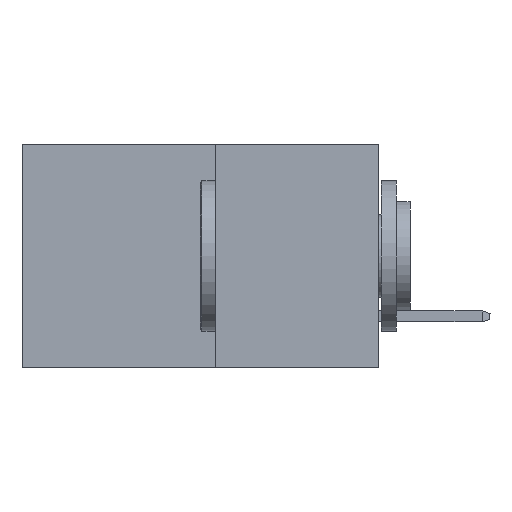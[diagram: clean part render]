
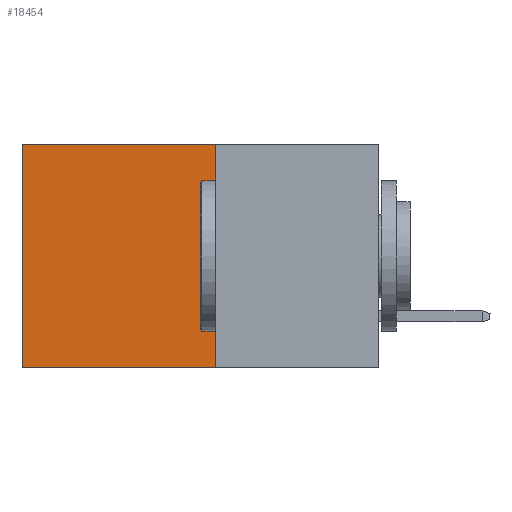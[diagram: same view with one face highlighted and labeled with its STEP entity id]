
A CAD part, left-side view. The second image highlights one B-rep face of the part: STEP entity #18454.
In plain terms, the highlighted planar face has unit normal (-1, 0, 0).
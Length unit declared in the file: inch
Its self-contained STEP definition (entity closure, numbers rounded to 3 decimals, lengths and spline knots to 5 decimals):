
#145 = CARTESIAN_POINT ( 'NONE',  ( 0.277, 0.59, -0.37 ) ) ;
#204 = VERTEX_POINT ( 'NONE', #19812 ) ;
#2008 = VECTOR ( 'NONE', #19218, 39.37008 ) ;
#2810 = LINE ( 'NONE', #18738, #2008 ) ;
#3067 = DIRECTION ( 'NONE',  ( 0., 0., -1. ) ) ;
#4759 = LINE ( 'NONE', #145, #11527 ) ;
#4954 = CARTESIAN_POINT ( 'NONE',  ( 0.277, 0.27, 0. ) ) ;
#6103 = ORIENTED_EDGE ( 'NONE', *, *, #27574, .F. ) ;
#7174 = ORIENTED_EDGE ( 'NONE', *, *, #7443, .T. ) ;
#7443 = EDGE_CURVE ( 'NONE', #14310, #204, #4759, .T. ) ;
#8168 = LINE ( 'NONE', #4954, #25371 ) ;
#8325 = CARTESIAN_POINT ( 'NONE',  ( 0.277, 0.59, 0. ) ) ;
#9046 = DIRECTION ( 'NONE',  ( 0., 1., 0. ) ) ;
#9050 = CARTESIAN_POINT ( 'NONE',  ( 0.277, 0.27, -0.37 ) ) ;
#9061 = EDGE_CURVE ( 'NONE', #31472, #10558, #2810, .T. ) ;
#10558 = VERTEX_POINT ( 'NONE', #24615 ) ;
#11527 = VECTOR ( 'NONE', #3067, 39.37008 ) ;
#11529 = EDGE_CURVE ( 'NONE', #31472, #14310, #8168, .T. ) ;
#11638 = DIRECTION ( 'NONE',  ( 1., 0., 0. ) ) ;
#11900 = AXIS2_PLACEMENT_3D ( 'NONE', #9050, #11638, #28634 ) ;
#12169 = ORIENTED_EDGE ( 'NONE', *, *, #9061, .F. ) ;
#14310 = VERTEX_POINT ( 'NONE', #8325 ) ;
#16032 = CARTESIAN_POINT ( 'NONE',  ( 0.277, 0.27, -0.37 ) ) ;
#16745 = FACE_OUTER_BOUND ( 'NONE', #29477, .T. ) ;
#18253 = LINE ( 'NONE', #16032, #29680 ) ;
#18402 = DIRECTION ( 'NONE',  ( 0., 1., 0. ) ) ;
#18454 = ADVANCED_FACE ( 'NONE', ( #16745 ), #23687, .F. ) ;
#18738 = CARTESIAN_POINT ( 'NONE',  ( 0.277, 0.27, -0.37 ) ) ;
#19218 = DIRECTION ( 'NONE',  ( 0., 0., -1. ) ) ;
#19812 = CARTESIAN_POINT ( 'NONE',  ( 0.277, 0.59, -0.37 ) ) ;
#23687 = PLANE ( 'NONE',  #11900 ) ;
#24615 = CARTESIAN_POINT ( 'NONE',  ( 0.277, 0.27, -0.37 ) ) ;
#25030 = ORIENTED_EDGE ( 'NONE', *, *, #11529, .T. ) ;
#25371 = VECTOR ( 'NONE', #9046, 39.37008 ) ;
#27574 = EDGE_CURVE ( 'NONE', #10558, #204, #18253, .T. ) ;
#28634 = DIRECTION ( 'NONE',  ( 0., 0., -1. ) ) ;
#29342 = CARTESIAN_POINT ( 'NONE',  ( 0.277, 0.27, 0. ) ) ;
#29477 = EDGE_LOOP ( 'NONE', ( #7174, #6103, #12169, #25030 ) ) ;
#29680 = VECTOR ( 'NONE', #18402, 39.37008 ) ;
#31472 = VERTEX_POINT ( 'NONE', #29342 ) ;
